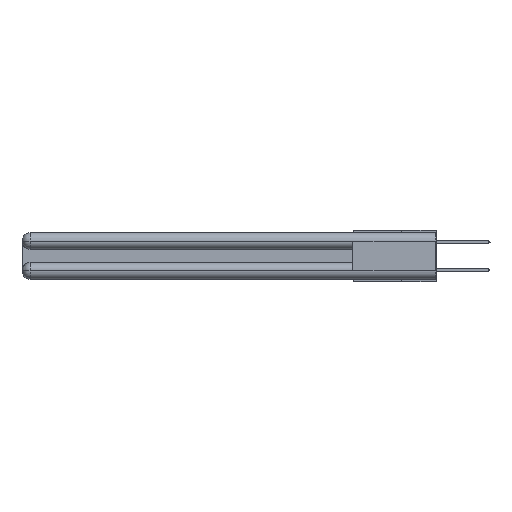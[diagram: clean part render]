
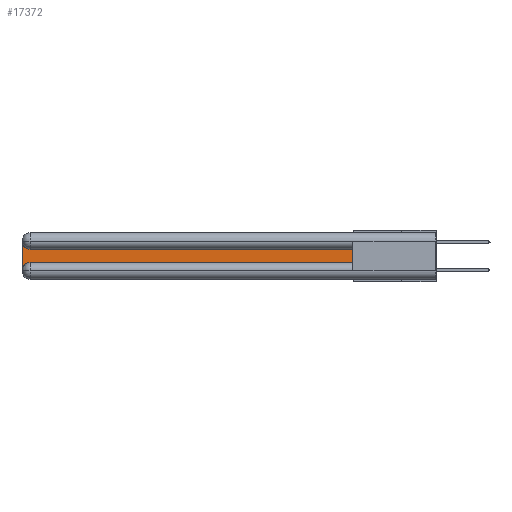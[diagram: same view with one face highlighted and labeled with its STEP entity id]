
A CAD part, left-side view. The second image highlights one B-rep face of the part: STEP entity #17372.
In plain terms, the highlighted planar face has unit normal (-1, 0, 0).
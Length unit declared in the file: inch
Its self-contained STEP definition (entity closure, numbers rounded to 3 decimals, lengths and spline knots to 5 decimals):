
#892 = ORIENTED_EDGE ( 'NONE', *, *, #8438, .T. ) ;
#1691 = FACE_OUTER_BOUND ( 'NONE', #6608, .T. ) ;
#1964 = EDGE_CURVE ( 'NONE', #10332, #16603, #15044, .T. ) ;
#2308 = EDGE_CURVE ( 'NONE', #11124, #20191, #9201, .T. ) ;
#3150 = DIRECTION ( 'NONE',  ( 0., -1., 0. ) ) ;
#3349 = VECTOR ( 'NONE', #21916, 39.37008 ) ;
#3828 = PLANE ( 'NONE',  #23489 ) ;
#3836 = CARTESIAN_POINT ( 'NONE',  ( 0.075, 0.6, -0.2175 ) ) ;
#4202 = CARTESIAN_POINT ( 'NONE',  ( 0.075, 3., -0.2175 ) ) ;
#4568 = CARTESIAN_POINT ( 'NONE',  ( 0.075, 0.6, -0.1225 ) ) ;
#4744 = LINE ( 'NONE', #3836, #24782 ) ;
#5816 = CARTESIAN_POINT ( 'NONE',  ( 0.075, 2.94, -0.0625 ) ) ;
#6324 = VERTEX_POINT ( 'NONE', #23748 ) ;
#6431 = DIRECTION ( 'NONE',  ( 1., 0., 0. ) ) ;
#6608 = EDGE_LOOP ( 'NONE', ( #11832, #10882, #17797, #17930, #892, #25197 ) ) ;
#7600 = AXIS2_PLACEMENT_3D ( 'NONE', #5816, #7972, #16844 ) ;
#7972 = DIRECTION ( 'NONE',  ( 1., 0., 0. ) ) ;
#7973 = AXIS2_PLACEMENT_3D ( 'NONE', #10837, #6431, #8605 ) ;
#8088 = EDGE_CURVE ( 'NONE', #6324, #21768, #4744, .T. ) ;
#8167 = DIRECTION ( 'NONE',  ( 0., 0., 1. ) ) ;
#8438 = EDGE_CURVE ( 'NONE', #16603, #6324, #15949, .T. ) ;
#8605 = DIRECTION ( 'NONE',  ( 0., 0., -1. ) ) ;
#9201 = CIRCLE ( 'NONE', #7600, 0.06 ) ;
#9380 = CARTESIAN_POINT ( 'NONE',  ( 0.075, 2.94, -0.2175 ) ) ;
#9790 = LINE ( 'NONE', #4202, #3349 ) ;
#10332 = VERTEX_POINT ( 'NONE', #15079 ) ;
#10837 = CARTESIAN_POINT ( 'NONE',  ( 0.075, 2.94, -0.2775 ) ) ;
#10882 = ORIENTED_EDGE ( 'NONE', *, *, #2308, .T. ) ;
#11124 = VERTEX_POINT ( 'NONE', #27146 ) ;
#11832 = ORIENTED_EDGE ( 'NONE', *, *, #13097, .T. ) ;
#12197 = VECTOR ( 'NONE', #3150, 39.37008 ) ;
#12348 = EDGE_CURVE ( 'NONE', #20191, #10332, #9790, .T. ) ;
#12657 = CARTESIAN_POINT ( 'NONE',  ( 0.075, 3., -0.1225 ) ) ;
#13097 = EDGE_CURVE ( 'NONE', #21768, #11124, #22996, .T. ) ;
#15044 = CIRCLE ( 'NONE', #7973, 0.06 ) ;
#15079 = CARTESIAN_POINT ( 'NONE',  ( 0.075, 3., -0.2775 ) ) ;
#15949 = LINE ( 'NONE', #20404, #12197 ) ;
#16603 = VERTEX_POINT ( 'NONE', #9380 ) ;
#16667 = DIRECTION ( 'NONE',  ( 1., 0., 0. ) ) ;
#16844 = DIRECTION ( 'NONE',  ( 0., 0., -1. ) ) ;
#17372 = ADVANCED_FACE ( 'NONE', ( #1691 ), #3828, .F. ) ;
#17797 = ORIENTED_EDGE ( 'NONE', *, *, #12348, .T. ) ;
#17930 = ORIENTED_EDGE ( 'NONE', *, *, #1964, .T. ) ;
#18724 = CARTESIAN_POINT ( 'NONE',  ( 0.075, 0.6, -0.1225 ) ) ;
#19545 = DIRECTION ( 'NONE',  ( 0., 1., 0. ) ) ;
#20191 = VERTEX_POINT ( 'NONE', #23907 ) ;
#20404 = CARTESIAN_POINT ( 'NONE',  ( 0.075, 0.6, -0.2175 ) ) ;
#21768 = VERTEX_POINT ( 'NONE', #18724 ) ;
#21916 = DIRECTION ( 'NONE',  ( 0., 0., -1. ) ) ;
#22996 = LINE ( 'NONE', #4568, #23677 ) ;
#23489 = AXIS2_PLACEMENT_3D ( 'NONE', #12657, #16667, #27860 ) ;
#23677 = VECTOR ( 'NONE', #19545, 39.37008 ) ;
#23748 = CARTESIAN_POINT ( 'NONE',  ( 0.075, 0.6, -0.2175 ) ) ;
#23907 = CARTESIAN_POINT ( 'NONE',  ( 0.075, 3., -0.0625 ) ) ;
#24782 = VECTOR ( 'NONE', #8167, 39.37008 ) ;
#25197 = ORIENTED_EDGE ( 'NONE', *, *, #8088, .T. ) ;
#27146 = CARTESIAN_POINT ( 'NONE',  ( 0.075, 2.94, -0.1225 ) ) ;
#27860 = DIRECTION ( 'NONE',  ( 0., 0., -1. ) ) ;
